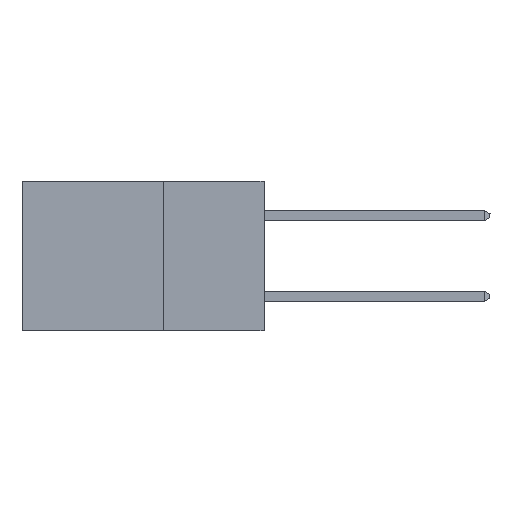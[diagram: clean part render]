
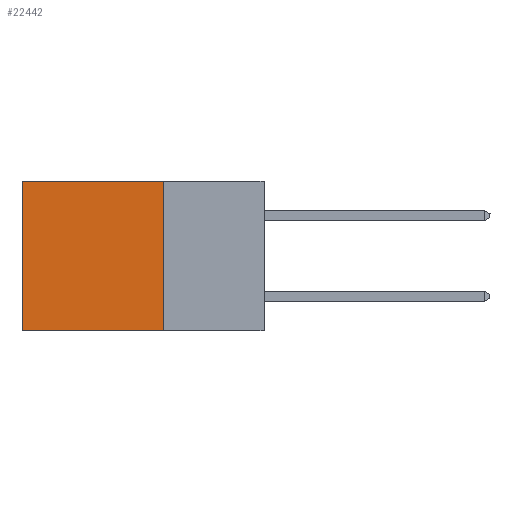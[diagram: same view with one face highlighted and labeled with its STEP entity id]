
A CAD part, left-side view. The second image highlights one B-rep face of the part: STEP entity #22442.
In plain terms, the highlighted planar face has unit normal (-1, 0, 0).
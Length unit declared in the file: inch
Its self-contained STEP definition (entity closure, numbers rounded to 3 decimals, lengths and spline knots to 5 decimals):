
#300 = VERTEX_POINT ( 'NONE', #23875 ) ;
#1072 = ORIENTED_EDGE ( 'NONE', *, *, #11780, .F. ) ;
#2660 = DIRECTION ( 'NONE',  ( 0., 0., -1. ) ) ;
#2961 = EDGE_LOOP ( 'NONE', ( #28701, #1072, #16091, #23126 ) ) ;
#3340 = LINE ( 'NONE', #12986, #10928 ) ;
#4004 = VECTOR ( 'NONE', #2660, 39.37008 ) ;
#4254 = EDGE_CURVE ( 'NONE', #13316, #15865, #3340, .T. ) ;
#8960 = DIRECTION ( 'NONE',  ( 0., 1., 0. ) ) ;
#9215 = VERTEX_POINT ( 'NONE', #11352 ) ;
#9915 = DIRECTION ( 'NONE',  ( 1., 0., 0. ) ) ;
#10928 = VECTOR ( 'NONE', #13080, 39.37008 ) ;
#11053 = EDGE_CURVE ( 'NONE', #15865, #300, #23681, .T. ) ;
#11352 = CARTESIAN_POINT ( 'NONE',  ( 0.298, 0.25, -0.37 ) ) ;
#11780 = EDGE_CURVE ( 'NONE', #9215, #300, #17984, .T. ) ;
#11917 = FACE_OUTER_BOUND ( 'NONE', #2961, .T. ) ;
#12316 = LINE ( 'NONE', #15074, #25143 ) ;
#12340 = DIRECTION ( 'NONE',  ( 0., 0., -1. ) ) ;
#12986 = CARTESIAN_POINT ( 'NONE',  ( 0.298, 0.25, 0. ) ) ;
#13080 = DIRECTION ( 'NONE',  ( 0., 1., 0. ) ) ;
#13316 = VERTEX_POINT ( 'NONE', #16570 ) ;
#13601 = CARTESIAN_POINT ( 'NONE',  ( 0.298, 0.25, -0.37 ) ) ;
#15074 = CARTESIAN_POINT ( 'NONE',  ( 0.298, 0.25, 0. ) ) ;
#15865 = VERTEX_POINT ( 'NONE', #26253 ) ;
#16091 = ORIENTED_EDGE ( 'NONE', *, *, #16659, .F. ) ;
#16570 = CARTESIAN_POINT ( 'NONE',  ( 0.298, 0.25, 0. ) ) ;
#16659 = EDGE_CURVE ( 'NONE', #13316, #9215, #12316, .T. ) ;
#17162 = CARTESIAN_POINT ( 'NONE',  ( 0.298, 0.6, 0. ) ) ;
#17541 = DIRECTION ( 'NONE',  ( 0., 0., -1. ) ) ;
#17984 = LINE ( 'NONE', #13601, #18330 ) ;
#18330 = VECTOR ( 'NONE', #8960, 39.37008 ) ;
#21984 = PLANE ( 'NONE',  #25635 ) ;
#22442 = ADVANCED_FACE ( 'NONE', ( #11917 ), #21984, .F. ) ;
#23126 = ORIENTED_EDGE ( 'NONE', *, *, #4254, .T. ) ;
#23681 = LINE ( 'NONE', #17162, #4004 ) ;
#23875 = CARTESIAN_POINT ( 'NONE',  ( 0.298, 0.6, -0.37 ) ) ;
#24404 = CARTESIAN_POINT ( 'NONE',  ( 0.298, 0.25, 0. ) ) ;
#25143 = VECTOR ( 'NONE', #17541, 39.37008 ) ;
#25635 = AXIS2_PLACEMENT_3D ( 'NONE', #24404, #9915, #12340 ) ;
#26253 = CARTESIAN_POINT ( 'NONE',  ( 0.298, 0.6, 0. ) ) ;
#28701 = ORIENTED_EDGE ( 'NONE', *, *, #11053, .T. ) ;
